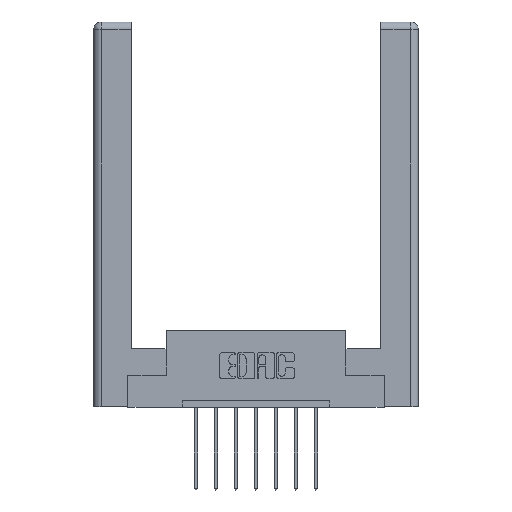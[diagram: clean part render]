
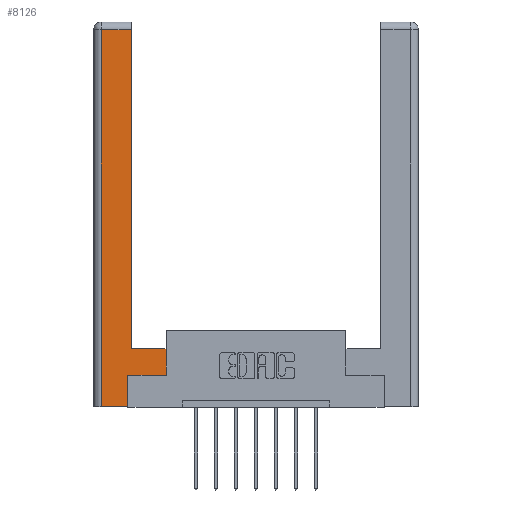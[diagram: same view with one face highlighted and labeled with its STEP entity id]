
A CAD part, top view. The second image highlights one B-rep face of the part: STEP entity #8126.
In plain terms, the highlighted planar face has unit normal (0, 0, 1).
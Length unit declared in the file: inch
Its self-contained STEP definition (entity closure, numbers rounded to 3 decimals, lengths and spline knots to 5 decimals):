
#250 = CARTESIAN_POINT ( 'NONE',  ( 0.295, 3., 0. ) ) ;
#499 = DIRECTION ( 'NONE',  ( 0., 0., -1. ) ) ;
#706 = VECTOR ( 'NONE', #3133, 39.37008 ) ;
#1017 = LINE ( 'NONE', #1819, #6138 ) ;
#1072 = ORIENTED_EDGE ( 'NONE', *, *, #11355, .T. ) ;
#1748 = LINE ( 'NONE', #250, #706 ) ;
#1795 = VERTEX_POINT ( 'NONE', #8345 ) ;
#1796 = CARTESIAN_POINT ( 'NONE',  ( 0.265, 0., 0. ) ) ;
#1819 = CARTESIAN_POINT ( 'NONE',  ( 0.0615, 2.94, 0. ) ) ;
#2323 = CARTESIAN_POINT ( 'NONE',  ( 0.0615, 2.94, 0. ) ) ;
#2325 = VECTOR ( 'NONE', #4295, 39.37008 ) ;
#2389 = CARTESIAN_POINT ( 'NONE',  ( 0.295, 2.94, 0. ) ) ;
#2480 = EDGE_CURVE ( 'NONE', #6190, #6925, #10567, .T. ) ;
#2713 = EDGE_CURVE ( 'NONE', #6925, #1795, #6990, .T. ) ;
#3133 = DIRECTION ( 'NONE',  ( 0., 1., 0. ) ) ;
#3165 = CARTESIAN_POINT ( 'NONE',  ( 0.265, 0.245, 0. ) ) ;
#3209 = DIRECTION ( 'NONE',  ( 0., 1., 0. ) ) ;
#3257 = CARTESIAN_POINT ( 'NONE',  ( 0.565, 0.45, 0. ) ) ;
#3406 = CARTESIAN_POINT ( 'NONE',  ( 0.565, 0.245, 0. ) ) ;
#3424 = ORIENTED_EDGE ( 'NONE', *, *, #6271, .T. ) ;
#3487 = AXIS2_PLACEMENT_3D ( 'NONE', #7332, #499, #12134 ) ;
#3600 = ORIENTED_EDGE ( 'NONE', *, *, #3841, .T. ) ;
#3811 = VERTEX_POINT ( 'NONE', #11827 ) ;
#3841 = EDGE_CURVE ( 'NONE', #11817, #7103, #8621, .T. ) ;
#4018 = VECTOR ( 'NONE', #3209, 39.37008 ) ;
#4139 = DIRECTION ( 'NONE',  ( -1., 0., 0. ) ) ;
#4295 = DIRECTION ( 'NONE',  ( 0., 1., 0. ) ) ;
#4398 = VECTOR ( 'NONE', #11286, 39.37008 ) ;
#4585 = DIRECTION ( 'NONE',  ( 0., -1., 0. ) ) ;
#4698 = LINE ( 'NONE', #9145, #6989 ) ;
#4868 = LINE ( 'NONE', #3257, #2325 ) ;
#4956 = ORIENTED_EDGE ( 'NONE', *, *, #8024, .T. ) ;
#5388 = VECTOR ( 'NONE', #11160, 39.37008 ) ;
#5821 = EDGE_LOOP ( 'NONE', ( #1072, #9792, #10227, #6929, #7047, #3600, #3424, #4956 ) ) ;
#5900 = FACE_OUTER_BOUND ( 'NONE', #5821, .T. ) ;
#6138 = VECTOR ( 'NONE', #11435, 39.37008 ) ;
#6190 = VERTEX_POINT ( 'NONE', #2323 ) ;
#6271 = EDGE_CURVE ( 'NONE', #7103, #8652, #4868, .T. ) ;
#6874 = CARTESIAN_POINT ( 'NONE',  ( 0.565, 0.245, 0. ) ) ;
#6925 = VERTEX_POINT ( 'NONE', #12195 ) ;
#6929 = ORIENTED_EDGE ( 'NONE', *, *, #2713, .T. ) ;
#6989 = VECTOR ( 'NONE', #4139, 39.37008 ) ;
#6990 = LINE ( 'NONE', #1796, #4398 ) ;
#7047 = ORIENTED_EDGE ( 'NONE', *, *, #11012, .T. ) ;
#7103 = VERTEX_POINT ( 'NONE', #6874 ) ;
#7286 = CARTESIAN_POINT ( 'NONE',  ( 0.565, 0.45, 0. ) ) ;
#7332 = CARTESIAN_POINT ( 'NONE',  ( 0., 0., 0. ) ) ;
#8024 = EDGE_CURVE ( 'NONE', #8652, #3811, #4698, .T. ) ;
#8126 = ADVANCED_FACE ( 'NONE', ( #5900 ), #12047, .F. ) ;
#8345 = CARTESIAN_POINT ( 'NONE',  ( 0.265, 0., 0. ) ) ;
#8621 = LINE ( 'NONE', #3406, #5388 ) ;
#8652 = VERTEX_POINT ( 'NONE', #7286 ) ;
#8740 = CARTESIAN_POINT ( 'NONE',  ( 0.265, 0.245, 0. ) ) ;
#8964 = VECTOR ( 'NONE', #4585, 39.37008 ) ;
#9145 = CARTESIAN_POINT ( 'NONE',  ( 0.295, 0.45, 0. ) ) ;
#9792 = ORIENTED_EDGE ( 'NONE', *, *, #10679, .T. ) ;
#9955 = VERTEX_POINT ( 'NONE', #2389 ) ;
#10227 = ORIENTED_EDGE ( 'NONE', *, *, #2480, .T. ) ;
#10360 = LINE ( 'NONE', #3165, #4018 ) ;
#10567 = LINE ( 'NONE', #12291, #8964 ) ;
#10679 = EDGE_CURVE ( 'NONE', #9955, #6190, #1017, .T. ) ;
#11012 = EDGE_CURVE ( 'NONE', #1795, #11817, #10360, .T. ) ;
#11160 = DIRECTION ( 'NONE',  ( 1., 0., 0. ) ) ;
#11286 = DIRECTION ( 'NONE',  ( 1., 0., 0. ) ) ;
#11355 = EDGE_CURVE ( 'NONE', #3811, #9955, #1748, .T. ) ;
#11435 = DIRECTION ( 'NONE',  ( -1., 0., 0. ) ) ;
#11817 = VERTEX_POINT ( 'NONE', #8740 ) ;
#11827 = CARTESIAN_POINT ( 'NONE',  ( 0.295, 0.45, 0. ) ) ;
#12047 = PLANE ( 'NONE',  #3487 ) ;
#12134 = DIRECTION ( 'NONE',  ( -1., 0., 0. ) ) ;
#12195 = CARTESIAN_POINT ( 'NONE',  ( 0.0615, 0., 0. ) ) ;
#12291 = CARTESIAN_POINT ( 'NONE',  ( 0.0615, 0., 0. ) ) ;
